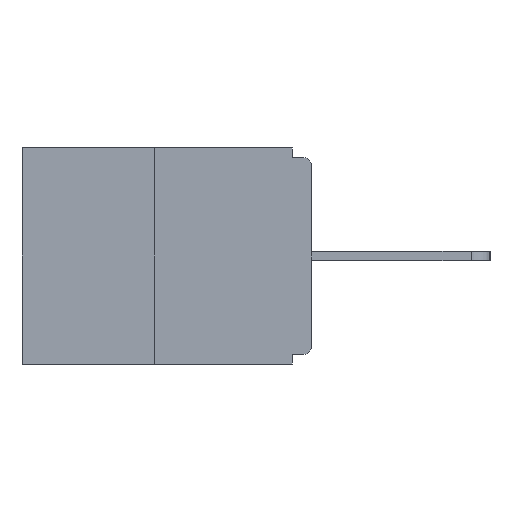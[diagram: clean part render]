
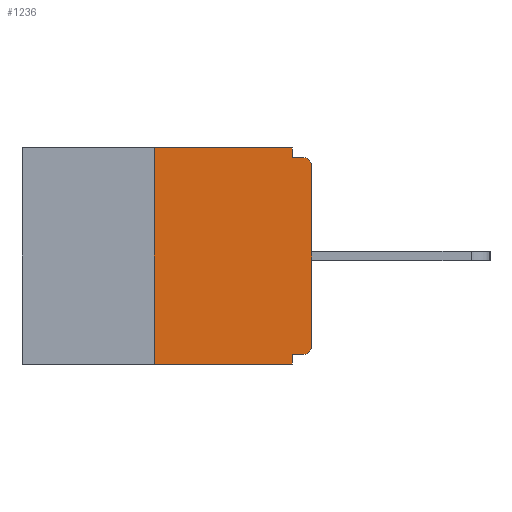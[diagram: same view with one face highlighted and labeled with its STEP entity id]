
A CAD part, left-side view. The second image highlights one B-rep face of the part: STEP entity #1236.
In plain terms, the highlighted planar face has unit normal (-1, 0, 0).
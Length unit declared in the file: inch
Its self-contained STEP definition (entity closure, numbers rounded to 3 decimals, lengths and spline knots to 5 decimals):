
#52 = ORIENTED_EDGE ( 'NONE', *, *, #17532, .T. ) ;
#226 = CIRCLE ( 'NONE', #2898, 0.015 ) ;
#305 = EDGE_CURVE ( 'NONE', #14885, #3603, #17774, .T. ) ;
#700 = CARTESIAN_POINT ( 'NONE',  ( 0., 0.25, 0. ) ) ;
#724 = ORIENTED_EDGE ( 'NONE', *, *, #1676, .F. ) ;
#754 = CARTESIAN_POINT ( 'NONE',  ( 0., 0.46, -0.343 ) ) ;
#821 = CARTESIAN_POINT ( 'NONE',  ( 0., 0.46, 0. ) ) ;
#833 = VECTOR ( 'NONE', #4131, 39.37008 ) ;
#994 = DIRECTION ( 'NONE',  ( 0., -1., 0. ) ) ;
#1037 = VERTEX_POINT ( 'NONE', #14707 ) ;
#1236 = ADVANCED_FACE ( 'NONE', ( #16661 ), #15014, .F. ) ;
#1286 = VECTOR ( 'NONE', #994, 39.37008 ) ;
#1538 = AXIS2_PLACEMENT_3D ( 'NONE', #19333, #6925, #7026 ) ;
#1676 = EDGE_CURVE ( 'NONE', #17193, #9598, #14896, .T. ) ;
#1744 = CARTESIAN_POINT ( 'NONE',  ( 0., 0., -0.328 ) ) ;
#1968 = ORIENTED_EDGE ( 'NONE', *, *, #12292, .F. ) ;
#2058 = DIRECTION ( 'NONE',  ( 0., 1., 0. ) ) ;
#2267 = LINE ( 'NONE', #5677, #5928 ) ;
#2426 = VECTOR ( 'NONE', #8731, 39.37008 ) ;
#2438 = LINE ( 'NONE', #754, #4636 ) ;
#2510 = DIRECTION ( 'NONE',  ( 1., 0., 0. ) ) ;
#2738 = EDGE_CURVE ( 'NONE', #17964, #8396, #226, .T. ) ;
#2881 = LINE ( 'NONE', #4444, #833 ) ;
#2898 = AXIS2_PLACEMENT_3D ( 'NONE', #8929, #15453, #16793 ) ;
#3038 = EDGE_CURVE ( 'NONE', #13899, #8396, #15870, .T. ) ;
#3184 = AXIS2_PLACEMENT_3D ( 'NONE', #821, #2510, #10461 ) ;
#3603 = VERTEX_POINT ( 'NONE', #4141 ) ;
#4131 = DIRECTION ( 'NONE',  ( 0., 0., -1. ) ) ;
#4141 = CARTESIAN_POINT ( 'NONE',  ( 0., 0.031, -0.328 ) ) ;
#4237 = CARTESIAN_POINT ( 'NONE',  ( 0., 0.46, 0. ) ) ;
#4444 = CARTESIAN_POINT ( 'NONE',  ( 0., 0.031, -0.343 ) ) ;
#4539 = VECTOR ( 'NONE', #18092, 39.37008 ) ;
#4636 = VECTOR ( 'NONE', #8543, 39.37008 ) ;
#4909 = ORIENTED_EDGE ( 'NONE', *, *, #6337, .T. ) ;
#5251 = EDGE_CURVE ( 'NONE', #9598, #1037, #8759, .T. ) ;
#5407 = ORIENTED_EDGE ( 'NONE', *, *, #2738, .T. ) ;
#5677 = CARTESIAN_POINT ( 'NONE',  ( 0., 0., 0. ) ) ;
#5707 = EDGE_CURVE ( 'NONE', #1037, #13899, #10590, .T. ) ;
#5928 = VECTOR ( 'NONE', #10318, 39.37008 ) ;
#6337 = EDGE_CURVE ( 'NONE', #14885, #11758, #11345, .T. ) ;
#6370 = CARTESIAN_POINT ( 'NONE',  ( 0., 0., -0.015 ) ) ;
#6925 = DIRECTION ( 'NONE',  ( -1., 0., 0. ) ) ;
#7026 = DIRECTION ( 'NONE',  ( 0., 0., -1. ) ) ;
#8396 = VERTEX_POINT ( 'NONE', #14173 ) ;
#8543 = DIRECTION ( 'NONE',  ( 0., -1., 0. ) ) ;
#8731 = DIRECTION ( 'NONE',  ( 0., 0., -1. ) ) ;
#8759 = LINE ( 'NONE', #4237, #1286 ) ;
#8929 = CARTESIAN_POINT ( 'NONE',  ( 0., 0.015, -0.03 ) ) ;
#9530 = CARTESIAN_POINT ( 'NONE',  ( 0., 0.25, 0. ) ) ;
#9598 = VERTEX_POINT ( 'NONE', #9530 ) ;
#10001 = ORIENTED_EDGE ( 'NONE', *, *, #5707, .F. ) ;
#10318 = DIRECTION ( 'NONE',  ( 0., 0., 1. ) ) ;
#10461 = DIRECTION ( 'NONE',  ( 0., 0., -1. ) ) ;
#10590 = LINE ( 'NONE', #18151, #2426 ) ;
#10736 = VECTOR ( 'NONE', #2058, 39.37008 ) ;
#11128 = ORIENTED_EDGE ( 'NONE', *, *, #3038, .F. ) ;
#11165 = CARTESIAN_POINT ( 'NONE',  ( 0., 0.031, -0.015 ) ) ;
#11345 = CIRCLE ( 'NONE', #1538, 0.015 ) ;
#11758 = VERTEX_POINT ( 'NONE', #17114 ) ;
#11885 = CARTESIAN_POINT ( 'NONE',  ( 0., 0.25, -0.343 ) ) ;
#12292 = EDGE_CURVE ( 'NONE', #3603, #16069, #2881, .T. ) ;
#12581 = ORIENTED_EDGE ( 'NONE', *, *, #18015, .T. ) ;
#13899 = VERTEX_POINT ( 'NONE', #11165 ) ;
#14173 = CARTESIAN_POINT ( 'NONE',  ( 0., 0.015, -0.015 ) ) ;
#14707 = CARTESIAN_POINT ( 'NONE',  ( 0., 0.031, 0. ) ) ;
#14885 = VERTEX_POINT ( 'NONE', #15667 ) ;
#14896 = LINE ( 'NONE', #700, #4539 ) ;
#14991 = CARTESIAN_POINT ( 'NONE',  ( 0., 0.031, -0.343 ) ) ;
#15014 = PLANE ( 'NONE',  #3184 ) ;
#15453 = DIRECTION ( 'NONE',  ( -1., 0., 0. ) ) ;
#15667 = CARTESIAN_POINT ( 'NONE',  ( 0., 0.015, -0.328 ) ) ;
#15870 = LINE ( 'NONE', #6370, #16544 ) ;
#16069 = VERTEX_POINT ( 'NONE', #14991 ) ;
#16292 = ORIENTED_EDGE ( 'NONE', *, *, #5251, .F. ) ;
#16466 = ORIENTED_EDGE ( 'NONE', *, *, #305, .F. ) ;
#16544 = VECTOR ( 'NONE', #19187, 39.37008 ) ;
#16661 = FACE_OUTER_BOUND ( 'NONE', #20059, .T. ) ;
#16793 = DIRECTION ( 'NONE',  ( 0., 0., -1. ) ) ;
#17114 = CARTESIAN_POINT ( 'NONE',  ( 0., 0., -0.313 ) ) ;
#17193 = VERTEX_POINT ( 'NONE', #11885 ) ;
#17532 = EDGE_CURVE ( 'NONE', #11758, #17964, #2267, .T. ) ;
#17774 = LINE ( 'NONE', #1744, #10736 ) ;
#17838 = CARTESIAN_POINT ( 'NONE',  ( 0., 0., -0.03 ) ) ;
#17964 = VERTEX_POINT ( 'NONE', #17838 ) ;
#18015 = EDGE_CURVE ( 'NONE', #17193, #16069, #2438, .T. ) ;
#18092 = DIRECTION ( 'NONE',  ( 0., 0., 1. ) ) ;
#18151 = CARTESIAN_POINT ( 'NONE',  ( 0., 0.031, 0. ) ) ;
#19187 = DIRECTION ( 'NONE',  ( 0., -1., 0. ) ) ;
#19333 = CARTESIAN_POINT ( 'NONE',  ( 0., 0.015, -0.313 ) ) ;
#20059 = EDGE_LOOP ( 'NONE', ( #16292, #724, #12581, #1968, #16466, #4909, #52, #5407, #11128, #10001 ) ) ;
